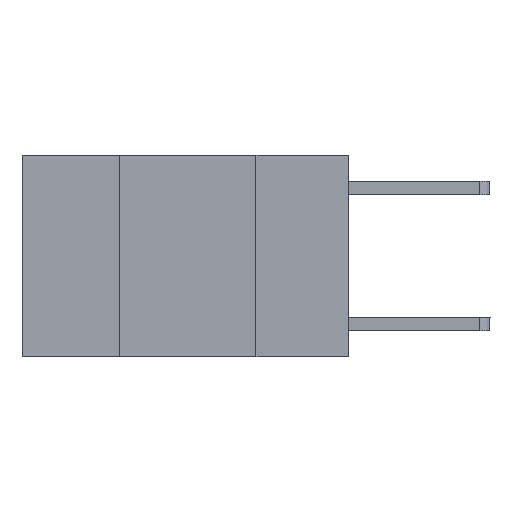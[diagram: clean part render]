
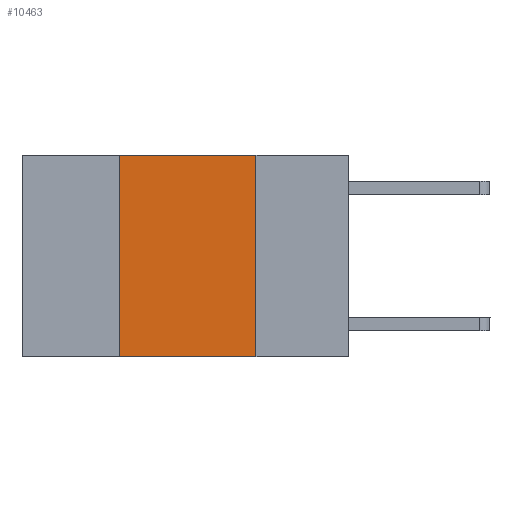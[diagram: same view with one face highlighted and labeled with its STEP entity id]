
A CAD part, left-side view. The second image highlights one B-rep face of the part: STEP entity #10463.
In plain terms, the highlighted planar face has unit normal (-1, 0, 0).
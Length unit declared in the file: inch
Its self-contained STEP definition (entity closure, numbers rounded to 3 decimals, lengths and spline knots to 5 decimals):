
#473 = DIRECTION ( 'NONE',  ( 0., 0., -1. ) ) ;
#1157 = EDGE_CURVE ( 'NONE', #3598, #10477, #5445, .T. ) ;
#1392 = LINE ( 'NONE', #4361, #8734 ) ;
#1800 = DIRECTION ( 'NONE',  ( 0., -1., 0. ) ) ;
#2393 = CARTESIAN_POINT ( 'NONE',  ( 0., 0.6, 0. ) ) ;
#2461 = DIRECTION ( 'NONE',  ( 0., 0., 1. ) ) ;
#2515 = VECTOR ( 'NONE', #1800, 39.37008 ) ;
#2605 = VECTOR ( 'NONE', #9576, 39.37008 ) ;
#2718 = CARTESIAN_POINT ( 'NONE',  ( 0., 0.17, -0.37 ) ) ;
#2831 = CARTESIAN_POINT ( 'NONE',  ( 0., 0.42, 0. ) ) ;
#3002 = CARTESIAN_POINT ( 'NONE',  ( 0., 0.42, -0.37 ) ) ;
#3451 = EDGE_CURVE ( 'NONE', #3598, #8948, #7608, .T. ) ;
#3598 = VERTEX_POINT ( 'NONE', #3002 ) ;
#3857 = CARTESIAN_POINT ( 'NONE',  ( 0., 0.17, 0. ) ) ;
#4091 = CARTESIAN_POINT ( 'NONE',  ( 0., 0.6, 0. ) ) ;
#4356 = PLANE ( 'NONE',  #11996 ) ;
#4361 = CARTESIAN_POINT ( 'NONE',  ( 0., 0.17, 0. ) ) ;
#5445 = LINE ( 'NONE', #2831, #7944 ) ;
#5636 = EDGE_CURVE ( 'NONE', #5956, #8948, #1392, .T. ) ;
#5956 = VERTEX_POINT ( 'NONE', #3857 ) ;
#6232 = FACE_OUTER_BOUND ( 'NONE', #6905, .T. ) ;
#6260 = DIRECTION ( 'NONE',  ( 1., 0., 0. ) ) ;
#6644 = EDGE_CURVE ( 'NONE', #10477, #5956, #9895, .T. ) ;
#6658 = ORIENTED_EDGE ( 'NONE', *, *, #5636, .F. ) ;
#6826 = ORIENTED_EDGE ( 'NONE', *, *, #6644, .F. ) ;
#6840 = ORIENTED_EDGE ( 'NONE', *, *, #1157, .F. ) ;
#6905 = EDGE_LOOP ( 'NONE', ( #6658, #6826, #6840, #7128 ) ) ;
#7128 = ORIENTED_EDGE ( 'NONE', *, *, #3451, .T. ) ;
#7608 = LINE ( 'NONE', #12171, #2515 ) ;
#7944 = VECTOR ( 'NONE', #2461, 39.37008 ) ;
#8734 = VECTOR ( 'NONE', #10013, 39.37008 ) ;
#8948 = VERTEX_POINT ( 'NONE', #2718 ) ;
#9576 = DIRECTION ( 'NONE',  ( 0., -1., 0. ) ) ;
#9895 = LINE ( 'NONE', #4091, #2605 ) ;
#10013 = DIRECTION ( 'NONE',  ( 0., 0., -1. ) ) ;
#10463 = ADVANCED_FACE ( 'NONE', ( #6232 ), #4356, .F. ) ;
#10477 = VERTEX_POINT ( 'NONE', #10994 ) ;
#10994 = CARTESIAN_POINT ( 'NONE',  ( 0., 0.42, 0. ) ) ;
#11996 = AXIS2_PLACEMENT_3D ( 'NONE', #2393, #6260, #473 ) ;
#12171 = CARTESIAN_POINT ( 'NONE',  ( 0., 0.6, -0.37 ) ) ;
